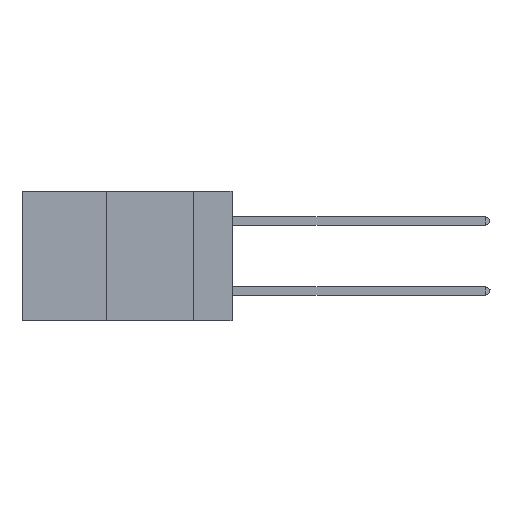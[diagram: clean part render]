
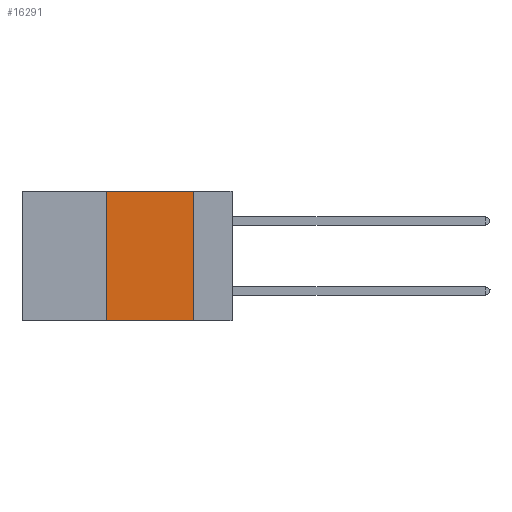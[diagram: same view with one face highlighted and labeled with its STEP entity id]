
A CAD part, left-side view. The second image highlights one B-rep face of the part: STEP entity #16291.
In plain terms, the highlighted planar face has unit normal (-1, 0, 0).
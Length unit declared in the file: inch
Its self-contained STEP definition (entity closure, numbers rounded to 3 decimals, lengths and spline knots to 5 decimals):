
#222 = EDGE_CURVE ( 'NONE', #15114, #8566, #8925, .T. ) ;
#403 = ORIENTED_EDGE ( 'NONE', *, *, #7906, .F. ) ;
#2115 = DIRECTION ( 'NONE',  ( 0., 0., 1. ) ) ;
#2903 = LINE ( 'NONE', #14511, #6429 ) ;
#3222 = CARTESIAN_POINT ( 'NONE',  ( 0., 0.36, 0. ) ) ;
#3690 = CARTESIAN_POINT ( 'NONE',  ( 0., 0.11, 0. ) ) ;
#3798 = VECTOR ( 'NONE', #7803, 39.37008 ) ;
#4154 = VECTOR ( 'NONE', #2115, 39.37008 ) ;
#4644 = DIRECTION ( 'NONE',  ( 0., -1., 0. ) ) ;
#4998 = CARTESIAN_POINT ( 'NONE',  ( 0., 0.36, 0. ) ) ;
#5120 = LINE ( 'NONE', #3690, #3798 ) ;
#5321 = ORIENTED_EDGE ( 'NONE', *, *, #9761, .F. ) ;
#5389 = FACE_OUTER_BOUND ( 'NONE', #10542, .T. ) ;
#6429 = VECTOR ( 'NONE', #4644, 39.37008 ) ;
#6676 = DIRECTION ( 'NONE',  ( 1., 0., 0. ) ) ;
#7803 = DIRECTION ( 'NONE',  ( 0., 0., -1. ) ) ;
#7906 = EDGE_CURVE ( 'NONE', #14274, #8566, #5120, .T. ) ;
#8119 = EDGE_CURVE ( 'NONE', #16358, #14274, #2903, .T. ) ;
#8309 = ORIENTED_EDGE ( 'NONE', *, *, #8119, .F. ) ;
#8566 = VERTEX_POINT ( 'NONE', #9003 ) ;
#8735 = LINE ( 'NONE', #4998, #4154 ) ;
#8925 = LINE ( 'NONE', #14697, #13939 ) ;
#9003 = CARTESIAN_POINT ( 'NONE',  ( 0., 0.11, -0.37 ) ) ;
#9197 = PLANE ( 'NONE',  #15434 ) ;
#9761 = EDGE_CURVE ( 'NONE', #15114, #16358, #8735, .T. ) ;
#10433 = ORIENTED_EDGE ( 'NONE', *, *, #222, .T. ) ;
#10542 = EDGE_LOOP ( 'NONE', ( #403, #8309, #5321, #10433 ) ) ;
#10592 = CARTESIAN_POINT ( 'NONE',  ( 0., 0.11, 0. ) ) ;
#12842 = CARTESIAN_POINT ( 'NONE',  ( 0., 0.36, -0.37 ) ) ;
#13939 = VECTOR ( 'NONE', #16065, 39.37008 ) ;
#14274 = VERTEX_POINT ( 'NONE', #10592 ) ;
#14511 = CARTESIAN_POINT ( 'NONE',  ( 0., 0.6, 0. ) ) ;
#14697 = CARTESIAN_POINT ( 'NONE',  ( 0., 0.6, -0.37 ) ) ;
#15015 = CARTESIAN_POINT ( 'NONE',  ( 0., 0.6, 0. ) ) ;
#15114 = VERTEX_POINT ( 'NONE', #12842 ) ;
#15184 = DIRECTION ( 'NONE',  ( 0., 0., -1. ) ) ;
#15434 = AXIS2_PLACEMENT_3D ( 'NONE', #15015, #6676, #15184 ) ;
#16065 = DIRECTION ( 'NONE',  ( 0., -1., 0. ) ) ;
#16291 = ADVANCED_FACE ( 'NONE', ( #5389 ), #9197, .F. ) ;
#16358 = VERTEX_POINT ( 'NONE', #3222 ) ;
